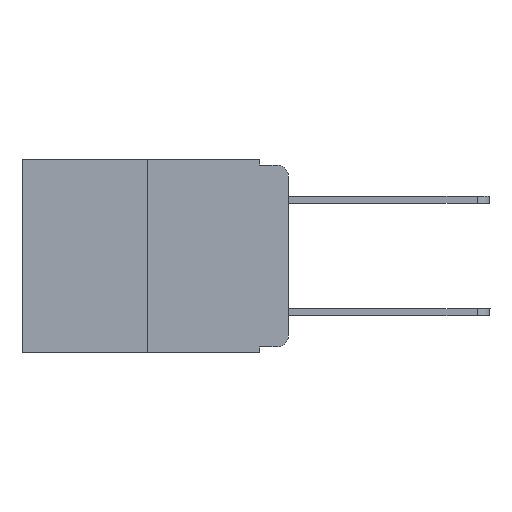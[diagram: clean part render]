
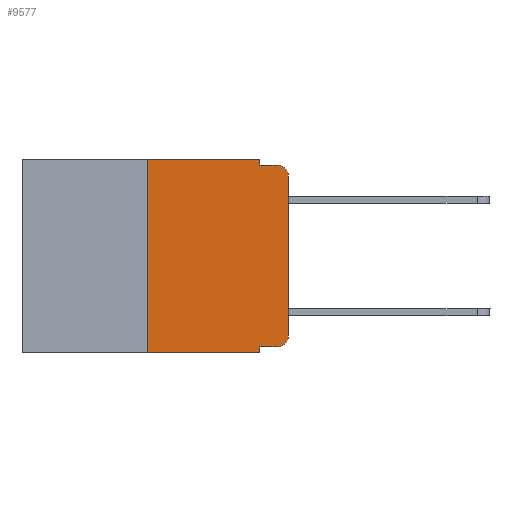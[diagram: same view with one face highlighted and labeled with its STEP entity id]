
A CAD part, left-side view. The second image highlights one B-rep face of the part: STEP entity #9577.
In plain terms, the highlighted planar face has unit normal (-1, 0, 0).
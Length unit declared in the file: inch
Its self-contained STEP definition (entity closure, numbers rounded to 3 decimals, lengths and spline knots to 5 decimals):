
#141 = ORIENTED_EDGE ( 'NONE', *, *, #4580, .F. ) ;
#585 = LINE ( 'NONE', #6623, #7492 ) ;
#1240 = ORIENTED_EDGE ( 'NONE', *, *, #14270, .F. ) ;
#1742 = CARTESIAN_POINT ( 'NONE',  ( 0., 0.051, 0. ) ) ;
#1827 = CIRCLE ( 'NONE', #6626, 0.02 ) ;
#2153 = VECTOR ( 'NONE', #10551, 39.37008 ) ;
#2269 = ORIENTED_EDGE ( 'NONE', *, *, #12891, .F. ) ;
#2336 = DIRECTION ( 'NONE',  ( 0., 0., -1. ) ) ;
#2559 = DIRECTION ( 'NONE',  ( 0., 0., 1. ) ) ;
#2587 = LINE ( 'NONE', #17309, #15509 ) ;
#2679 = CIRCLE ( 'NONE', #16543, 0.02 ) ;
#2687 = VERTEX_POINT ( 'NONE', #6613 ) ;
#2690 = DIRECTION ( 'NONE',  ( -1., 0., 0. ) ) ;
#3311 = DIRECTION ( 'NONE',  ( 0., 0., -1. ) ) ;
#3511 = CARTESIAN_POINT ( 'NONE',  ( 0., 0.25, 0. ) ) ;
#3521 = LINE ( 'NONE', #14789, #14473 ) ;
#3702 = EDGE_CURVE ( 'NONE', #14186, #16787, #10578, .T. ) ;
#3981 = VECTOR ( 'NONE', #5096, 39.37008 ) ;
#4190 = LINE ( 'NONE', #9191, #3981 ) ;
#4192 = CARTESIAN_POINT ( 'NONE',  ( 0., 0.02, -0.333 ) ) ;
#4580 = EDGE_CURVE ( 'NONE', #13719, #16787, #2587, .T. ) ;
#4843 = ORIENTED_EDGE ( 'NONE', *, *, #3702, .T. ) ;
#4893 = ORIENTED_EDGE ( 'NONE', *, *, #8479, .T. ) ;
#5096 = DIRECTION ( 'NONE',  ( 0., -1., 0. ) ) ;
#5192 = EDGE_CURVE ( 'NONE', #14186, #10970, #8378, .T. ) ;
#5255 = CARTESIAN_POINT ( 'NONE',  ( 0., 0.25, 0. ) ) ;
#5286 = LINE ( 'NONE', #16392, #17559 ) ;
#5507 = VERTEX_POINT ( 'NONE', #6226 ) ;
#6226 = CARTESIAN_POINT ( 'NONE',  ( 0., 0., -0.313 ) ) ;
#6247 = EDGE_LOOP ( 'NONE', ( #16070, #10661, #1240, #6393, #2269, #13631, #4843, #141, #12325, #4893 ) ) ;
#6347 = DIRECTION ( 'NONE',  ( -1., 0., 0. ) ) ;
#6393 = ORIENTED_EDGE ( 'NONE', *, *, #15678, .F. ) ;
#6457 = EDGE_CURVE ( 'NONE', #5507, #12231, #585, .T. ) ;
#6613 = CARTESIAN_POINT ( 'NONE',  ( 0., 0.051, -0.01 ) ) ;
#6623 = CARTESIAN_POINT ( 'NONE',  ( 0., 0., 0. ) ) ;
#6626 = AXIS2_PLACEMENT_3D ( 'NONE', #15204, #2690, #12305 ) ;
#6713 = DIRECTION ( 'NONE',  ( 0., 0., -1. ) ) ;
#7492 = VECTOR ( 'NONE', #16288, 39.37008 ) ;
#7675 = DIRECTION ( 'NONE',  ( 0., 0., -1. ) ) ;
#7792 = CARTESIAN_POINT ( 'NONE',  ( 0., 0.051, -0.343 ) ) ;
#8026 = EDGE_CURVE ( 'NONE', #13719, #12811, #4190, .T. ) ;
#8137 = CARTESIAN_POINT ( 'NONE',  ( 0., 0.02, -0.01 ) ) ;
#8378 = LINE ( 'NONE', #5255, #16312 ) ;
#8479 = EDGE_CURVE ( 'NONE', #12811, #5507, #2679, .T. ) ;
#9076 = CARTESIAN_POINT ( 'NONE',  ( 0., 0., -0.03 ) ) ;
#9163 = CARTESIAN_POINT ( 'NONE',  ( 0., 0.473, -0.343 ) ) ;
#9191 = CARTESIAN_POINT ( 'NONE',  ( 0., 0.051, -0.333 ) ) ;
#9196 = DIRECTION ( 'NONE',  ( 0., -1., 0. ) ) ;
#9577 = ADVANCED_FACE ( 'NONE', ( #14639 ), #14239, .F. ) ;
#9735 = DIRECTION ( 'NONE',  ( 0., -1., 0. ) ) ;
#10109 = CARTESIAN_POINT ( 'NONE',  ( 0., 0.051, 0. ) ) ;
#10121 = VERTEX_POINT ( 'NONE', #10109 ) ;
#10180 = CARTESIAN_POINT ( 'NONE',  ( 0., 0.473, 0. ) ) ;
#10551 = DIRECTION ( 'NONE',  ( 0., -1., 0. ) ) ;
#10578 = LINE ( 'NONE', #9163, #2153 ) ;
#10621 = CARTESIAN_POINT ( 'NONE',  ( 0., 0.02, -0.313 ) ) ;
#10639 = CARTESIAN_POINT ( 'NONE',  ( 0., 0.25, -0.343 ) ) ;
#10661 = ORIENTED_EDGE ( 'NONE', *, *, #16311, .T. ) ;
#10970 = VERTEX_POINT ( 'NONE', #3511 ) ;
#11340 = VECTOR ( 'NONE', #6713, 39.37008 ) ;
#11885 = VERTEX_POINT ( 'NONE', #8137 ) ;
#12231 = VERTEX_POINT ( 'NONE', #9076 ) ;
#12305 = DIRECTION ( 'NONE',  ( 0., 0., -1. ) ) ;
#12325 = ORIENTED_EDGE ( 'NONE', *, *, #8026, .T. ) ;
#12811 = VERTEX_POINT ( 'NONE', #4192 ) ;
#12891 = EDGE_CURVE ( 'NONE', #10970, #10121, #5286, .T. ) ;
#13631 = ORIENTED_EDGE ( 'NONE', *, *, #5192, .F. ) ;
#13719 = VERTEX_POINT ( 'NONE', #15425 ) ;
#14186 = VERTEX_POINT ( 'NONE', #10639 ) ;
#14239 = PLANE ( 'NONE',  #15766 ) ;
#14270 = EDGE_CURVE ( 'NONE', #2687, #11885, #3521, .T. ) ;
#14473 = VECTOR ( 'NONE', #9196, 39.37008 ) ;
#14639 = FACE_OUTER_BOUND ( 'NONE', #6247, .T. ) ;
#14789 = CARTESIAN_POINT ( 'NONE',  ( 0., 0.051, -0.01 ) ) ;
#15204 = CARTESIAN_POINT ( 'NONE',  ( 0., 0.02, -0.03 ) ) ;
#15425 = CARTESIAN_POINT ( 'NONE',  ( 0., 0.051, -0.333 ) ) ;
#15509 = VECTOR ( 'NONE', #2336, 39.37008 ) ;
#15663 = LINE ( 'NONE', #1742, #11340 ) ;
#15678 = EDGE_CURVE ( 'NONE', #10121, #2687, #15663, .T. ) ;
#15766 = AXIS2_PLACEMENT_3D ( 'NONE', #10180, #16961, #3311 ) ;
#16070 = ORIENTED_EDGE ( 'NONE', *, *, #6457, .T. ) ;
#16288 = DIRECTION ( 'NONE',  ( 0., 0., 1. ) ) ;
#16311 = EDGE_CURVE ( 'NONE', #12231, #11885, #1827, .T. ) ;
#16312 = VECTOR ( 'NONE', #2559, 39.37008 ) ;
#16392 = CARTESIAN_POINT ( 'NONE',  ( 0., 0.473, 0. ) ) ;
#16543 = AXIS2_PLACEMENT_3D ( 'NONE', #10621, #6347, #7675 ) ;
#16787 = VERTEX_POINT ( 'NONE', #7792 ) ;
#16961 = DIRECTION ( 'NONE',  ( 1., 0., 0. ) ) ;
#17309 = CARTESIAN_POINT ( 'NONE',  ( 0., 0.051, 0. ) ) ;
#17559 = VECTOR ( 'NONE', #9735, 39.37008 ) ;
